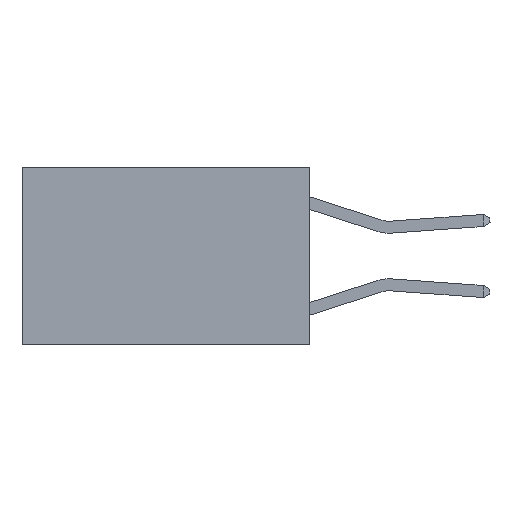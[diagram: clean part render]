
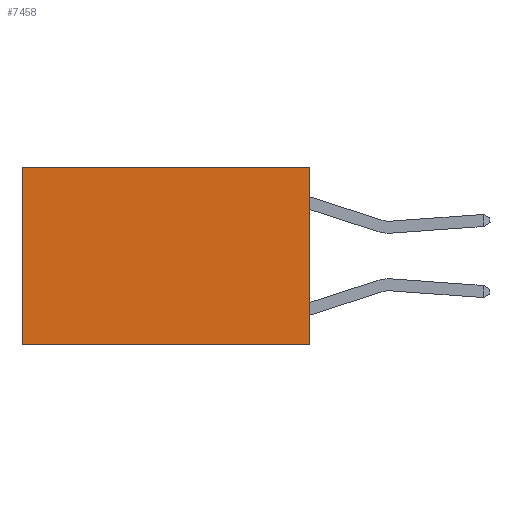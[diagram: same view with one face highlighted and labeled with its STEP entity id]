
A CAD part, left-side view. The second image highlights one B-rep face of the part: STEP entity #7458.
In plain terms, the highlighted planar face has unit normal (-1, 0, 0).
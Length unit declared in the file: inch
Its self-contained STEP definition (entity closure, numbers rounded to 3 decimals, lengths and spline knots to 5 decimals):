
#156 = LINE ( 'NONE', #2452, #8428 ) ;
#191 = ORIENTED_EDGE ( 'NONE', *, *, #5960, .T. ) ;
#665 = FACE_OUTER_BOUND ( 'NONE', #2267, .T. ) ;
#1210 = ORIENTED_EDGE ( 'NONE', *, *, #2232, .F. ) ;
#1427 = DIRECTION ( 'NONE',  ( 0., 1., 0. ) ) ;
#1520 = CARTESIAN_POINT ( 'NONE',  ( 0.2625, 0., -0.37 ) ) ;
#2232 = EDGE_CURVE ( 'NONE', #7202, #12805, #4046, .T. ) ;
#2267 = EDGE_LOOP ( 'NONE', ( #4575, #1210, #4260, #191 ) ) ;
#2452 = CARTESIAN_POINT ( 'NONE',  ( 0.2625, 0.6, 0. ) ) ;
#2540 = CARTESIAN_POINT ( 'NONE',  ( 0.2625, 0., 0. ) ) ;
#3126 = CARTESIAN_POINT ( 'NONE',  ( 0.2625, 0., 0. ) ) ;
#3217 = CARTESIAN_POINT ( 'NONE',  ( 0.2625, 0., 0. ) ) ;
#3561 = CARTESIAN_POINT ( 'NONE',  ( 0.2625, 0.6, 0. ) ) ;
#4046 = LINE ( 'NONE', #1520, #12156 ) ;
#4260 = ORIENTED_EDGE ( 'NONE', *, *, #5250, .F. ) ;
#4575 = ORIENTED_EDGE ( 'NONE', *, *, #12990, .T. ) ;
#4723 = AXIS2_PLACEMENT_3D ( 'NONE', #3126, #11558, #5188 ) ;
#5188 = DIRECTION ( 'NONE',  ( 0., 0., -1. ) ) ;
#5250 = EDGE_CURVE ( 'NONE', #9611, #7202, #9360, .T. ) ;
#5960 = EDGE_CURVE ( 'NONE', #9611, #11798, #8520, .T. ) ;
#6064 = VECTOR ( 'NONE', #7970, 39.37008 ) ;
#6822 = DIRECTION ( 'NONE',  ( 0., 1., 0. ) ) ;
#7202 = VERTEX_POINT ( 'NONE', #7820 ) ;
#7458 = ADVANCED_FACE ( 'NONE', ( #665 ), #10542, .F. ) ;
#7820 = CARTESIAN_POINT ( 'NONE',  ( 0.2625, 0., -0.37 ) ) ;
#7970 = DIRECTION ( 'NONE',  ( 0., 0., -1. ) ) ;
#8428 = VECTOR ( 'NONE', #11920, 39.37008 ) ;
#8520 = LINE ( 'NONE', #2540, #13702 ) ;
#9360 = LINE ( 'NONE', #13155, #6064 ) ;
#9611 = VERTEX_POINT ( 'NONE', #3217 ) ;
#10542 = PLANE ( 'NONE',  #4723 ) ;
#11558 = DIRECTION ( 'NONE',  ( 1., 0., 0. ) ) ;
#11798 = VERTEX_POINT ( 'NONE', #3561 ) ;
#11920 = DIRECTION ( 'NONE',  ( 0., 0., -1. ) ) ;
#12156 = VECTOR ( 'NONE', #6822, 39.37008 ) ;
#12745 = CARTESIAN_POINT ( 'NONE',  ( 0.2625, 0.6, -0.37 ) ) ;
#12805 = VERTEX_POINT ( 'NONE', #12745 ) ;
#12990 = EDGE_CURVE ( 'NONE', #11798, #12805, #156, .T. ) ;
#13155 = CARTESIAN_POINT ( 'NONE',  ( 0.2625, 0., 0. ) ) ;
#13702 = VECTOR ( 'NONE', #1427, 39.37008 ) ;
